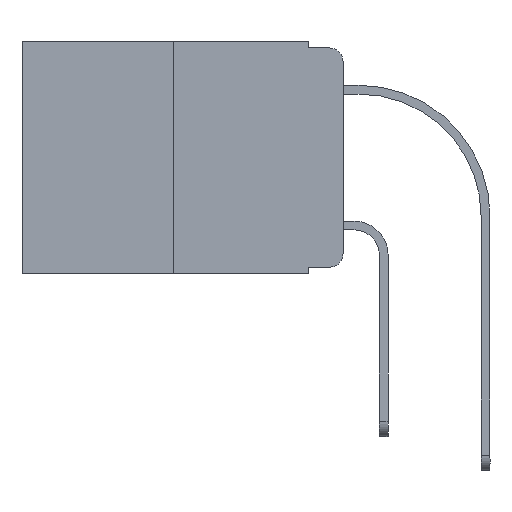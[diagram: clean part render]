
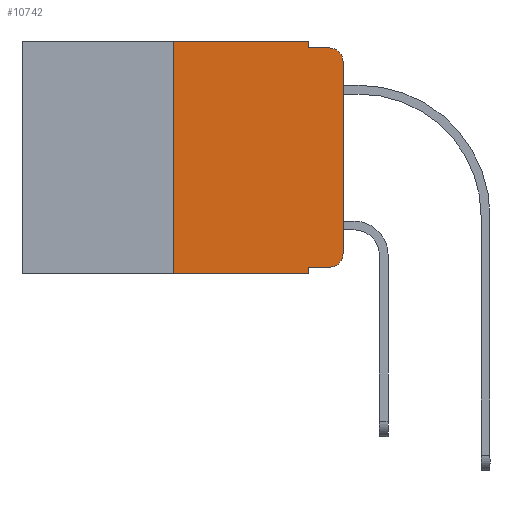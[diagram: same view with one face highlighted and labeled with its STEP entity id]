
A CAD part, left-side view. The second image highlights one B-rep face of the part: STEP entity #10742.
In plain terms, the highlighted planar face has unit normal (-1, 0, 0).
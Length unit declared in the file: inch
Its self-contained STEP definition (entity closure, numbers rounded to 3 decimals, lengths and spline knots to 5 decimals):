
#297 = DIRECTION ( 'NONE',  ( -1., 0., 0. ) ) ;
#353 = CARTESIAN_POINT ( 'NONE',  ( 0., 0.473, 0. ) ) ;
#426 = DIRECTION ( 'NONE',  ( 0., 0., -1. ) ) ;
#464 = EDGE_CURVE ( 'NONE', #2405, #7119, #10523, .T. ) ;
#533 = ORIENTED_EDGE ( 'NONE', *, *, #11192, .T. ) ;
#571 = VERTEX_POINT ( 'NONE', #3923 ) ;
#748 = VERTEX_POINT ( 'NONE', #2737 ) ;
#1271 = CARTESIAN_POINT ( 'NONE',  ( 0., 0.473, 0. ) ) ;
#1371 = CIRCLE ( 'NONE', #8391, 0.02 ) ;
#1463 = LINE ( 'NONE', #12200, #2575 ) ;
#1718 = PLANE ( 'NONE',  #2801 ) ;
#1778 = CARTESIAN_POINT ( 'NONE',  ( 0., 0.25, -0.343 ) ) ;
#1791 = CARTESIAN_POINT ( 'NONE',  ( 0., 0.051, -0.01 ) ) ;
#2154 = EDGE_LOOP ( 'NONE', ( #533, #3403, #8522, #10701, #2281, #6014, #10105, #3244, #6407, #4559 ) ) ;
#2271 = DIRECTION ( 'NONE',  ( 0., -1., 0. ) ) ;
#2281 = ORIENTED_EDGE ( 'NONE', *, *, #3948, .F. ) ;
#2405 = VERTEX_POINT ( 'NONE', #9399 ) ;
#2546 = EDGE_CURVE ( 'NONE', #2405, #5505, #2643, .T. ) ;
#2575 = VECTOR ( 'NONE', #11126, 39.37008 ) ;
#2613 = DIRECTION ( 'NONE',  ( -1., 0., 0. ) ) ;
#2643 = LINE ( 'NONE', #3514, #9124 ) ;
#2658 = EDGE_CURVE ( 'NONE', #3345, #6131, #6417, .T. ) ;
#2725 = VECTOR ( 'NONE', #12329, 39.37008 ) ;
#2737 = CARTESIAN_POINT ( 'NONE',  ( 0., 0., -0.03 ) ) ;
#2801 = AXIS2_PLACEMENT_3D ( 'NONE', #353, #6084, #5132 ) ;
#3143 = CARTESIAN_POINT ( 'NONE',  ( 0., 0.25, 0. ) ) ;
#3209 = DIRECTION ( 'NONE',  ( 0., 0., 1. ) ) ;
#3244 = ORIENTED_EDGE ( 'NONE', *, *, #464, .F. ) ;
#3283 = LINE ( 'NONE', #5056, #12309 ) ;
#3345 = VERTEX_POINT ( 'NONE', #1791 ) ;
#3373 = CARTESIAN_POINT ( 'NONE',  ( 0., 0.02, -0.313 ) ) ;
#3403 = ORIENTED_EDGE ( 'NONE', *, *, #7097, .T. ) ;
#3514 = CARTESIAN_POINT ( 'NONE',  ( 0., 0.051, -0.333 ) ) ;
#3923 = CARTESIAN_POINT ( 'NONE',  ( 0., 0.25, 0. ) ) ;
#3948 = EDGE_CURVE ( 'NONE', #571, #5912, #7922, .T. ) ;
#4559 = ORIENTED_EDGE ( 'NONE', *, *, #8293, .T. ) ;
#4691 = DIRECTION ( 'NONE',  ( 0., -1., 0. ) ) ;
#4794 = EDGE_CURVE ( 'NONE', #5912, #3345, #3283, .T. ) ;
#5056 = CARTESIAN_POINT ( 'NONE',  ( 0., 0.051, 0. ) ) ;
#5059 = EDGE_CURVE ( 'NONE', #11335, #7119, #5632, .T. ) ;
#5132 = DIRECTION ( 'NONE',  ( 0., 0., -1. ) ) ;
#5505 = VERTEX_POINT ( 'NONE', #6594 ) ;
#5632 = LINE ( 'NONE', #11488, #9469 ) ;
#5912 = VERTEX_POINT ( 'NONE', #9330 ) ;
#5965 = VECTOR ( 'NONE', #2271, 39.37008 ) ;
#5969 = AXIS2_PLACEMENT_3D ( 'NONE', #9216, #2613, #8338 ) ;
#5987 = VECTOR ( 'NONE', #8389, 39.37008 ) ;
#6014 = ORIENTED_EDGE ( 'NONE', *, *, #6527, .F. ) ;
#6084 = DIRECTION ( 'NONE',  ( 1., 0., 0. ) ) ;
#6131 = VERTEX_POINT ( 'NONE', #10896 ) ;
#6407 = ORIENTED_EDGE ( 'NONE', *, *, #2546, .T. ) ;
#6417 = LINE ( 'NONE', #8432, #2725 ) ;
#6514 = CARTESIAN_POINT ( 'NONE',  ( 0., 0.051, -0.343 ) ) ;
#6527 = EDGE_CURVE ( 'NONE', #11335, #571, #10934, .T. ) ;
#6594 = CARTESIAN_POINT ( 'NONE',  ( 0., 0.02, -0.333 ) ) ;
#6773 = VECTOR ( 'NONE', #3209, 39.37008 ) ;
#7097 = EDGE_CURVE ( 'NONE', #748, #6131, #10789, .T. ) ;
#7119 = VERTEX_POINT ( 'NONE', #6514 ) ;
#7922 = LINE ( 'NONE', #1271, #5965 ) ;
#8293 = EDGE_CURVE ( 'NONE', #5505, #9073, #1371, .T. ) ;
#8338 = DIRECTION ( 'NONE',  ( 0., 0., -1. ) ) ;
#8389 = DIRECTION ( 'NONE',  ( 0., 0., -1. ) ) ;
#8391 = AXIS2_PLACEMENT_3D ( 'NONE', #3373, #297, #426 ) ;
#8432 = CARTESIAN_POINT ( 'NONE',  ( 0., 0.051, -0.01 ) ) ;
#8461 = CARTESIAN_POINT ( 'NONE',  ( 0., 0.051, 0. ) ) ;
#8522 = ORIENTED_EDGE ( 'NONE', *, *, #2658, .F. ) ;
#9073 = VERTEX_POINT ( 'NONE', #11481 ) ;
#9124 = VECTOR ( 'NONE', #10371, 39.37008 ) ;
#9216 = CARTESIAN_POINT ( 'NONE',  ( 0., 0.02, -0.03 ) ) ;
#9316 = FACE_OUTER_BOUND ( 'NONE', #2154, .T. ) ;
#9330 = CARTESIAN_POINT ( 'NONE',  ( 0., 0.051, 0. ) ) ;
#9399 = CARTESIAN_POINT ( 'NONE',  ( 0., 0.051, -0.333 ) ) ;
#9469 = VECTOR ( 'NONE', #4691, 39.37008 ) ;
#9897 = DIRECTION ( 'NONE',  ( 0., 0., -1. ) ) ;
#10105 = ORIENTED_EDGE ( 'NONE', *, *, #5059, .T. ) ;
#10371 = DIRECTION ( 'NONE',  ( 0., -1., 0. ) ) ;
#10523 = LINE ( 'NONE', #8461, #5987 ) ;
#10701 = ORIENTED_EDGE ( 'NONE', *, *, #4794, .F. ) ;
#10742 = ADVANCED_FACE ( 'NONE', ( #9316 ), #1718, .F. ) ;
#10789 = CIRCLE ( 'NONE', #5969, 0.02 ) ;
#10896 = CARTESIAN_POINT ( 'NONE',  ( 0., 0.02, -0.01 ) ) ;
#10934 = LINE ( 'NONE', #3143, #6773 ) ;
#11126 = DIRECTION ( 'NONE',  ( 0., 0., 1. ) ) ;
#11192 = EDGE_CURVE ( 'NONE', #9073, #748, #1463, .T. ) ;
#11335 = VERTEX_POINT ( 'NONE', #1778 ) ;
#11481 = CARTESIAN_POINT ( 'NONE',  ( 0., 0., -0.313 ) ) ;
#11488 = CARTESIAN_POINT ( 'NONE',  ( 0., 0.473, -0.343 ) ) ;
#12200 = CARTESIAN_POINT ( 'NONE',  ( 0., 0., 0. ) ) ;
#12309 = VECTOR ( 'NONE', #9897, 39.37008 ) ;
#12329 = DIRECTION ( 'NONE',  ( 0., -1., 0. ) ) ;
